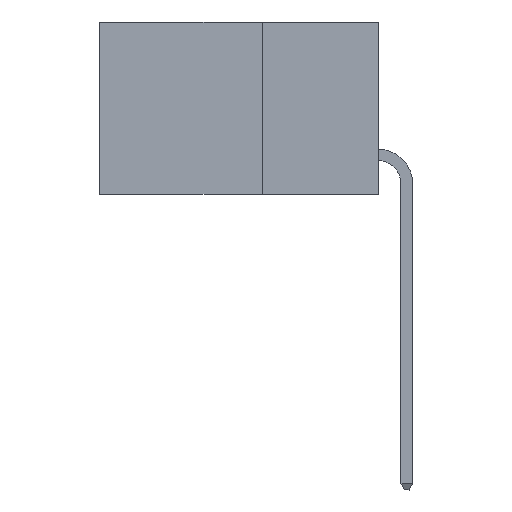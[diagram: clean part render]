
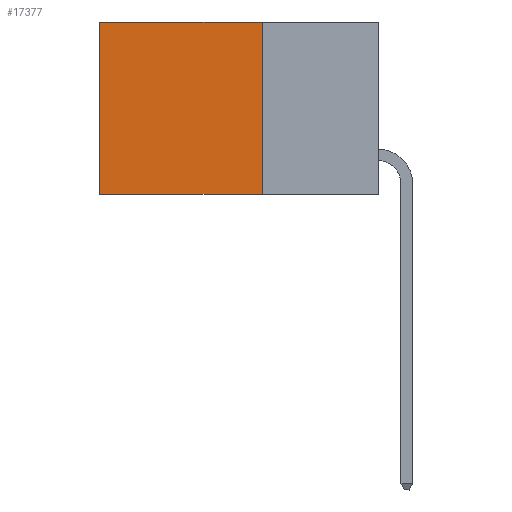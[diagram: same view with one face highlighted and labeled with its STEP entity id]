
A CAD part, left-side view. The second image highlights one B-rep face of the part: STEP entity #17377.
In plain terms, the highlighted planar face has unit normal (-1, 0, 0).
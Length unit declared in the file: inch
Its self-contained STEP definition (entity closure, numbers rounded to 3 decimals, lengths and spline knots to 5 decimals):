
#470 = DIRECTION ( 'NONE',  ( 0., 1., 0. ) ) ;
#3256 = EDGE_CURVE ( 'NONE', #5005, #15093, #23630, .T. ) ;
#3317 = CARTESIAN_POINT ( 'NONE',  ( 0.2615, 0.25, -0.37 ) ) ;
#3449 = ORIENTED_EDGE ( 'NONE', *, *, #14100, .F. ) ;
#5005 = VERTEX_POINT ( 'NONE', #11435 ) ;
#5644 = CARTESIAN_POINT ( 'NONE',  ( 0.2615, 0.25, 0. ) ) ;
#5733 = DIRECTION ( 'NONE',  ( 0., 0., -1. ) ) ;
#7221 = PLANE ( 'NONE',  #8408 ) ;
#7862 = LINE ( 'NONE', #5644, #22920 ) ;
#7943 = EDGE_LOOP ( 'NONE', ( #16220, #14271, #3449, #18370 ) ) ;
#8408 = AXIS2_PLACEMENT_3D ( 'NONE', #24075, #20253, #14594 ) ;
#8929 = FACE_OUTER_BOUND ( 'NONE', #7943, .T. ) ;
#9863 = CARTESIAN_POINT ( 'NONE',  ( 0.2615, 0.25, 0. ) ) ;
#11435 = CARTESIAN_POINT ( 'NONE',  ( 0.2615, 0.25, -0.37 ) ) ;
#11808 = CARTESIAN_POINT ( 'NONE',  ( 0.2615, 0.6, -0.37 ) ) ;
#12709 = VECTOR ( 'NONE', #5733, 39.37008 ) ;
#13481 = CARTESIAN_POINT ( 'NONE',  ( 0.2615, 0.25, -0.37 ) ) ;
#13614 = EDGE_CURVE ( 'NONE', #24120, #23517, #7862, .T. ) ;
#14100 = EDGE_CURVE ( 'NONE', #24120, #5005, #18796, .T. ) ;
#14185 = LINE ( 'NONE', #23553, #19510 ) ;
#14271 = ORIENTED_EDGE ( 'NONE', *, *, #3256, .F. ) ;
#14594 = DIRECTION ( 'NONE',  ( 0., 0., -1. ) ) ;
#15093 = VERTEX_POINT ( 'NONE', #11808 ) ;
#16220 = ORIENTED_EDGE ( 'NONE', *, *, #21952, .T. ) ;
#17377 = ADVANCED_FACE ( 'NONE', ( #8929 ), #7221, .F. ) ;
#17767 = VECTOR ( 'NONE', #19685, 39.37008 ) ;
#18258 = DIRECTION ( 'NONE',  ( 0., 0., -1. ) ) ;
#18370 = ORIENTED_EDGE ( 'NONE', *, *, #13614, .T. ) ;
#18796 = LINE ( 'NONE', #13481, #12709 ) ;
#19510 = VECTOR ( 'NONE', #18258, 39.37008 ) ;
#19685 = DIRECTION ( 'NONE',  ( 0., 1., 0. ) ) ;
#20253 = DIRECTION ( 'NONE',  ( 1., 0., 0. ) ) ;
#21115 = CARTESIAN_POINT ( 'NONE',  ( 0.2615, 0.6, 0. ) ) ;
#21952 = EDGE_CURVE ( 'NONE', #23517, #15093, #14185, .T. ) ;
#22920 = VECTOR ( 'NONE', #470, 39.37008 ) ;
#23517 = VERTEX_POINT ( 'NONE', #21115 ) ;
#23553 = CARTESIAN_POINT ( 'NONE',  ( 0.2615, 0.6, -0.37 ) ) ;
#23630 = LINE ( 'NONE', #3317, #17767 ) ;
#24075 = CARTESIAN_POINT ( 'NONE',  ( 0.2615, 0.25, -0.37 ) ) ;
#24120 = VERTEX_POINT ( 'NONE', #9863 ) ;
